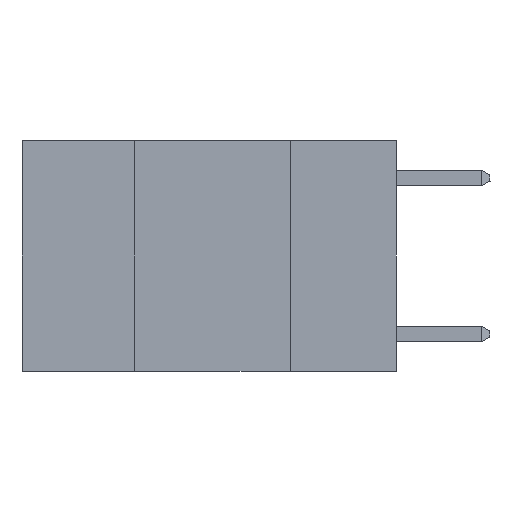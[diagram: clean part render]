
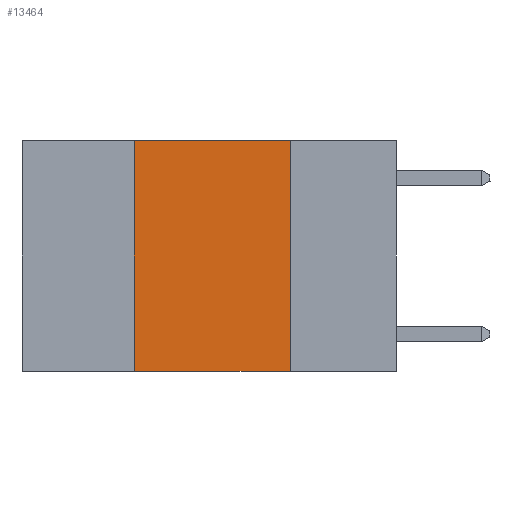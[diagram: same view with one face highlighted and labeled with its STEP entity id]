
A CAD part, left-side view. The second image highlights one B-rep face of the part: STEP entity #13464.
In plain terms, the highlighted planar face has unit normal (-1, 0, 0).
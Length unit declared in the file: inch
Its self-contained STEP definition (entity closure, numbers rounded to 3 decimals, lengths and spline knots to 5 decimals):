
#237 = CARTESIAN_POINT ( 'NONE',  ( 0., 0.17, -0.37 ) ) ;
#773 = ORIENTED_EDGE ( 'NONE', *, *, #23884, .F. ) ;
#1657 = ORIENTED_EDGE ( 'NONE', *, *, #7213, .T. ) ;
#1728 = CARTESIAN_POINT ( 'NONE',  ( 0., 0.6, -0.37 ) ) ;
#1882 = ORIENTED_EDGE ( 'NONE', *, *, #20551, .F. ) ;
#2134 = VECTOR ( 'NONE', #18653, 39.37008 ) ;
#2773 = CARTESIAN_POINT ( 'NONE',  ( 0., 0.42, -0.37 ) ) ;
#3674 = VERTEX_POINT ( 'NONE', #237 ) ;
#3771 = VERTEX_POINT ( 'NONE', #11149 ) ;
#4074 = FACE_OUTER_BOUND ( 'NONE', #14906, .T. ) ;
#4508 = VECTOR ( 'NONE', #21784, 39.37008 ) ;
#4664 = VECTOR ( 'NONE', #18225, 39.37008 ) ;
#4936 = CARTESIAN_POINT ( 'NONE',  ( 0., 0.6, 0. ) ) ;
#5169 = LINE ( 'NONE', #19697, #4508 ) ;
#7213 = EDGE_CURVE ( 'NONE', #15064, #3674, #8482, .T. ) ;
#7395 = VERTEX_POINT ( 'NONE', #17123 ) ;
#8482 = LINE ( 'NONE', #1728, #2134 ) ;
#11149 = CARTESIAN_POINT ( 'NONE',  ( 0., 0.17, 0. ) ) ;
#12457 = CARTESIAN_POINT ( 'NONE',  ( 0., 0.6, 0. ) ) ;
#13267 = LINE ( 'NONE', #4936, #24227 ) ;
#13464 = ADVANCED_FACE ( 'NONE', ( #4074 ), #24804, .F. ) ;
#14571 = DIRECTION ( 'NONE',  ( 0., 0., -1. ) ) ;
#14906 = EDGE_LOOP ( 'NONE', ( #773, #18603, #1882, #1657 ) ) ;
#15064 = VERTEX_POINT ( 'NONE', #2773 ) ;
#17123 = CARTESIAN_POINT ( 'NONE',  ( 0., 0.42, 0. ) ) ;
#18225 = DIRECTION ( 'NONE',  ( 0., 0., -1. ) ) ;
#18603 = ORIENTED_EDGE ( 'NONE', *, *, #19339, .F. ) ;
#18653 = DIRECTION ( 'NONE',  ( 0., -1., 0. ) ) ;
#19339 = EDGE_CURVE ( 'NONE', #7395, #3771, #13267, .T. ) ;
#19697 = CARTESIAN_POINT ( 'NONE',  ( 0., 0.42, 0. ) ) ;
#19703 = DIRECTION ( 'NONE',  ( 0., -1., 0. ) ) ;
#20551 = EDGE_CURVE ( 'NONE', #15064, #7395, #5169, .T. ) ;
#21486 = LINE ( 'NONE', #26318, #4664 ) ;
#21784 = DIRECTION ( 'NONE',  ( 0., 0., 1. ) ) ;
#23884 = EDGE_CURVE ( 'NONE', #3771, #3674, #21486, .T. ) ;
#23953 = AXIS2_PLACEMENT_3D ( 'NONE', #12457, #26824, #14571 ) ;
#24227 = VECTOR ( 'NONE', #19703, 39.37008 ) ;
#24804 = PLANE ( 'NONE',  #23953 ) ;
#26318 = CARTESIAN_POINT ( 'NONE',  ( 0., 0.17, 0. ) ) ;
#26824 = DIRECTION ( 'NONE',  ( 1., 0., 0. ) ) ;
